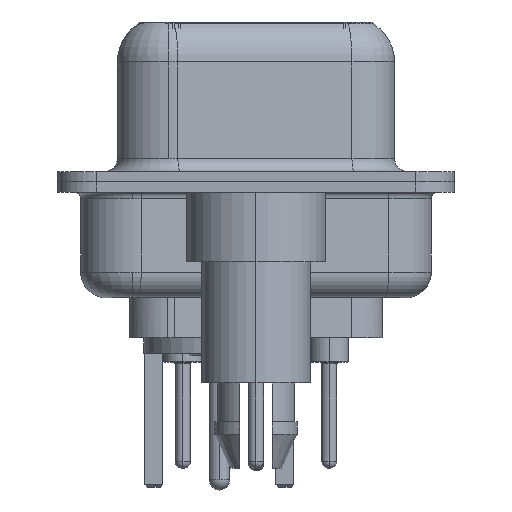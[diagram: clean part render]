
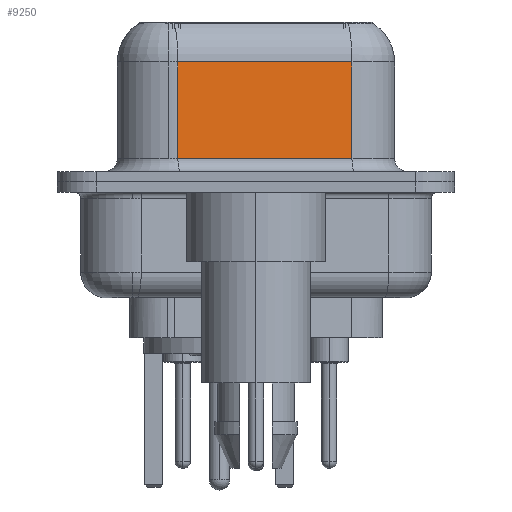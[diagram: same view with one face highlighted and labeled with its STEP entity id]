
A CAD part, left-side view. The second image highlights one B-rep face of the part: STEP entity #9250.
In plain terms, the highlighted planar face has unit normal (-0.985, -0.174, 0).
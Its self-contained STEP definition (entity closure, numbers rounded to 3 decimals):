
#2710 = ORIENTED_EDGE ( 'NONE', *, *, #15249, .T. ) ;
#3984 = AXIS2_PLACEMENT_3D ( 'NONE', #36096, #27788, #19655 ) ;
#5161 = ORIENTED_EDGE ( 'NONE', *, *, #6262, .T. ) ;
#5509 = VECTOR ( 'NONE', #17283, 1000. ) ;
#6262 = EDGE_CURVE ( 'NONE', #21462, #11570, #11451, .T. ) ;
#7218 = EDGE_LOOP ( 'NONE', ( #23669, #20918, #5161, #2710 ) ) ;
#7812 = DIRECTION ( 'NONE',  ( 0.174, -0.985, 0. ) ) ;
#9219 = CARTESIAN_POINT ( 'NONE',  ( 4.43, 3.028, 0.9 ) ) ;
#9250 = ADVANCED_FACE ( 'NONE', ( #34663 ), #13669, .F. ) ;
#11451 = LINE ( 'NONE', #16478, #19801 ) ;
#11570 = VERTEX_POINT ( 'NONE', #9219 ) ;
#11787 = VECTOR ( 'NONE', #32793, 1000. ) ;
#13669 = PLANE ( 'NONE',  #3984 ) ;
#13836 = VERTEX_POINT ( 'NONE', #29749 ) ;
#14359 = VECTOR ( 'NONE', #7812, 1000. ) ;
#15249 = EDGE_CURVE ( 'NONE', #11570, #32558, #20961, .T. ) ;
#16478 = CARTESIAN_POINT ( 'NONE',  ( 4.43, 3.028, 6.4 ) ) ;
#17283 = DIRECTION ( 'NONE',  ( 0., 0., -1. ) ) ;
#17807 = LINE ( 'NONE', #25794, #5509 ) ;
#19655 = DIRECTION ( 'NONE',  ( -0.174, 0.985, 0. ) ) ;
#19801 = VECTOR ( 'NONE', #27679, 1000. ) ;
#20918 = ORIENTED_EDGE ( 'NONE', *, *, #31849, .T. ) ;
#20961 = LINE ( 'NONE', #24653, #14359 ) ;
#21462 = VERTEX_POINT ( 'NONE', #24801 ) ;
#23669 = ORIENTED_EDGE ( 'NONE', *, *, #33853, .F. ) ;
#24653 = CARTESIAN_POINT ( 'NONE',  ( 5.621, -3.722, 0.9 ) ) ;
#24801 = CARTESIAN_POINT ( 'NONE',  ( 4.43, 3.028, 4.65 ) ) ;
#24995 = LINE ( 'NONE', #30484, #11787 ) ;
#25794 = CARTESIAN_POINT ( 'NONE',  ( 5.621, -3.722, 6.4 ) ) ;
#27679 = DIRECTION ( 'NONE',  ( 0., 0., -1. ) ) ;
#27788 = DIRECTION ( 'NONE',  ( 0.985, 0.174, 0. ) ) ;
#29749 = CARTESIAN_POINT ( 'NONE',  ( 5.621, -3.722, 4.65 ) ) ;
#30484 = CARTESIAN_POINT ( 'NONE',  ( 5.621, -3.722, 4.65 ) ) ;
#31849 = EDGE_CURVE ( 'NONE', #13836, #21462, #24995, .T. ) ;
#32558 = VERTEX_POINT ( 'NONE', #33320 ) ;
#32793 = DIRECTION ( 'NONE',  ( -0.174, 0.985, 0. ) ) ;
#33320 = CARTESIAN_POINT ( 'NONE',  ( 5.621, -3.722, 0.9 ) ) ;
#33853 = EDGE_CURVE ( 'NONE', #13836, #32558, #17807, .T. ) ;
#34663 = FACE_OUTER_BOUND ( 'NONE', #7218, .T. ) ;
#36096 = CARTESIAN_POINT ( 'NONE',  ( 5.621, -3.722, 6.4 ) ) ;
